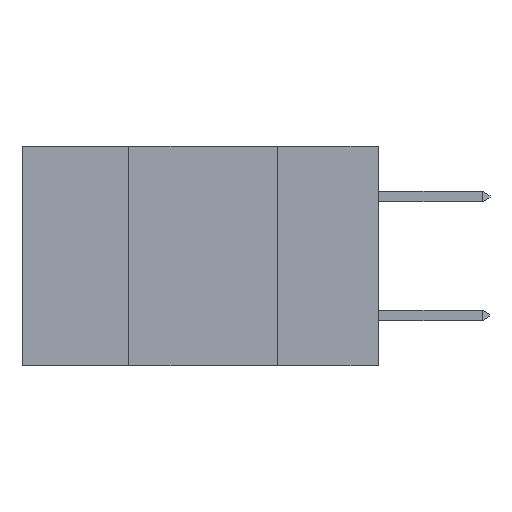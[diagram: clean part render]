
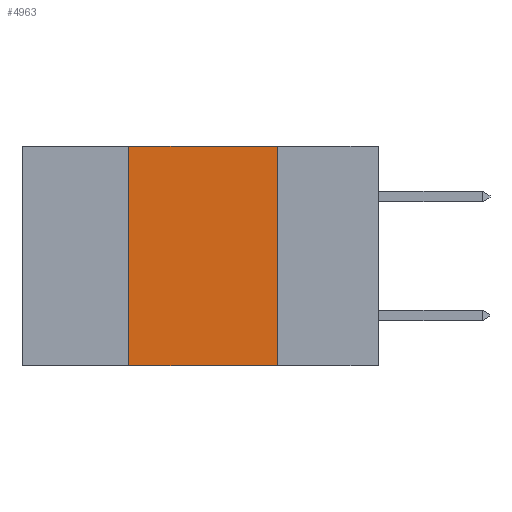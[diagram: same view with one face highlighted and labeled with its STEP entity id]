
A CAD part, left-side view. The second image highlights one B-rep face of the part: STEP entity #4963.
In plain terms, the highlighted planar face has unit normal (-1, 0, 0).
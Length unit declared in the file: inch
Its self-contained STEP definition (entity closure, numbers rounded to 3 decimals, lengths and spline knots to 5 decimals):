
#170 = DIRECTION ( 'NONE',  ( 0., -1., 0. ) ) ;
#338 = CARTESIAN_POINT ( 'NONE',  ( 0., 0.6, 0. ) ) ;
#568 = CARTESIAN_POINT ( 'NONE',  ( 0., 0.42, 0. ) ) ;
#1383 = VECTOR ( 'NONE', #3477, 39.37008 ) ;
#1772 = CARTESIAN_POINT ( 'NONE',  ( 0., 0.42, 0. ) ) ;
#2087 = LINE ( 'NONE', #568, #9839 ) ;
#2364 = DIRECTION ( 'NONE',  ( 0., 0., -1. ) ) ;
#2711 = EDGE_CURVE ( 'NONE', #12117, #3905, #5877, .T. ) ;
#3477 = DIRECTION ( 'NONE',  ( 0., -1., 0. ) ) ;
#3798 = DIRECTION ( 'NONE',  ( 0., 0., 1. ) ) ;
#3905 = VERTEX_POINT ( 'NONE', #12596 ) ;
#4049 = PLANE ( 'NONE',  #9746 ) ;
#4227 = LINE ( 'NONE', #7617, #1383 ) ;
#4392 = ORIENTED_EDGE ( 'NONE', *, *, #6521, .F. ) ;
#4612 = VERTEX_POINT ( 'NONE', #1772 ) ;
#4963 = ADVANCED_FACE ( 'NONE', ( #7928 ), #4049, .F. ) ;
#5195 = VECTOR ( 'NONE', #5422, 39.37008 ) ;
#5315 = ORIENTED_EDGE ( 'NONE', *, *, #8456, .T. ) ;
#5422 = DIRECTION ( 'NONE',  ( 0., 0., -1. ) ) ;
#5475 = CARTESIAN_POINT ( 'NONE',  ( 0., 0.17, 0. ) ) ;
#5877 = LINE ( 'NONE', #5475, #5195 ) ;
#6521 = EDGE_CURVE ( 'NONE', #4612, #12117, #4227, .T. ) ;
#6557 = CARTESIAN_POINT ( 'NONE',  ( 0., 0.6, -0.37 ) ) ;
#6976 = LINE ( 'NONE', #6557, #11307 ) ;
#7617 = CARTESIAN_POINT ( 'NONE',  ( 0., 0.6, 0. ) ) ;
#7928 = FACE_OUTER_BOUND ( 'NONE', #9339, .T. ) ;
#8456 = EDGE_CURVE ( 'NONE', #12718, #3905, #6976, .T. ) ;
#8501 = ORIENTED_EDGE ( 'NONE', *, *, #11345, .F. ) ;
#9204 = CARTESIAN_POINT ( 'NONE',  ( 0., 0.42, -0.37 ) ) ;
#9339 = EDGE_LOOP ( 'NONE', ( #10489, #4392, #8501, #5315 ) ) ;
#9746 = AXIS2_PLACEMENT_3D ( 'NONE', #338, #12793, #2364 ) ;
#9839 = VECTOR ( 'NONE', #3798, 39.37008 ) ;
#10349 = CARTESIAN_POINT ( 'NONE',  ( 0., 0.17, 0. ) ) ;
#10489 = ORIENTED_EDGE ( 'NONE', *, *, #2711, .F. ) ;
#11307 = VECTOR ( 'NONE', #170, 39.37008 ) ;
#11345 = EDGE_CURVE ( 'NONE', #12718, #4612, #2087, .T. ) ;
#12117 = VERTEX_POINT ( 'NONE', #10349 ) ;
#12596 = CARTESIAN_POINT ( 'NONE',  ( 0., 0.17, -0.37 ) ) ;
#12718 = VERTEX_POINT ( 'NONE', #9204 ) ;
#12793 = DIRECTION ( 'NONE',  ( 1., 0., 0. ) ) ;
